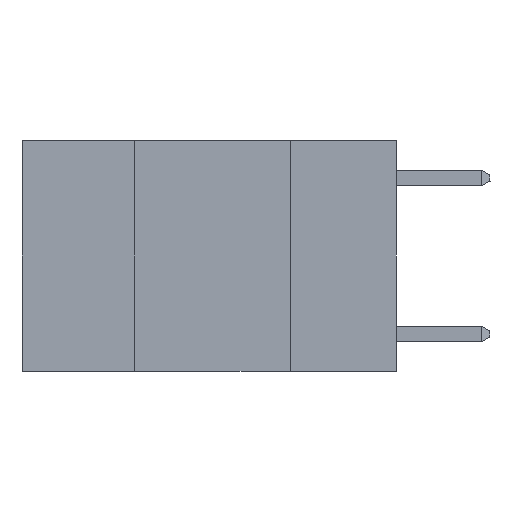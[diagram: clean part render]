
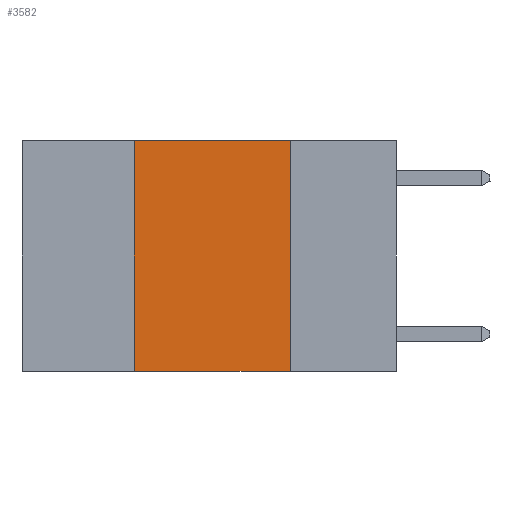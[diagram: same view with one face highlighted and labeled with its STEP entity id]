
A CAD part, left-side view. The second image highlights one B-rep face of the part: STEP entity #3582.
In plain terms, the highlighted planar face has unit normal (-1, 0, 0).
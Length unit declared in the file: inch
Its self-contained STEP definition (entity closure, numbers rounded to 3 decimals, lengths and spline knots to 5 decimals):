
#300 = DIRECTION ( 'NONE',  ( 0., -1., 0. ) ) ;
#587 = FACE_OUTER_BOUND ( 'NONE', #14649, .T. ) ;
#629 = AXIS2_PLACEMENT_3D ( 'NONE', #3977, #5288, #14118 ) ;
#1463 = LINE ( 'NONE', #1867, #2280 ) ;
#1574 = CARTESIAN_POINT ( 'NONE',  ( 0., 0.17, 0. ) ) ;
#1658 = VECTOR ( 'NONE', #9283, 39.37008 ) ;
#1867 = CARTESIAN_POINT ( 'NONE',  ( 0., 0.6, -0.37 ) ) ;
#2241 = LINE ( 'NONE', #16173, #15320 ) ;
#2280 = VECTOR ( 'NONE', #10849, 39.37008 ) ;
#2402 = VERTEX_POINT ( 'NONE', #11813 ) ;
#2422 = EDGE_CURVE ( 'NONE', #2402, #5420, #4739, .T. ) ;
#3582 = ADVANCED_FACE ( 'NONE', ( #587 ), #14069, .F. ) ;
#3977 = CARTESIAN_POINT ( 'NONE',  ( 0., 0.6, 0. ) ) ;
#4165 = CARTESIAN_POINT ( 'NONE',  ( 0., 0.42, 0. ) ) ;
#4739 = LINE ( 'NONE', #4165, #1658 ) ;
#5288 = DIRECTION ( 'NONE',  ( 1., 0., 0. ) ) ;
#5302 = CARTESIAN_POINT ( 'NONE',  ( 0., 0.42, 0. ) ) ;
#5420 = VERTEX_POINT ( 'NONE', #5302 ) ;
#6089 = LINE ( 'NONE', #9290, #15658 ) ;
#6255 = VERTEX_POINT ( 'NONE', #13141 ) ;
#6276 = DIRECTION ( 'NONE',  ( 0., 0., -1. ) ) ;
#8712 = EDGE_CURVE ( 'NONE', #16042, #6255, #2241, .T. ) ;
#9283 = DIRECTION ( 'NONE',  ( 0., 0., 1. ) ) ;
#9290 = CARTESIAN_POINT ( 'NONE',  ( 0., 0.6, 0. ) ) ;
#9646 = EDGE_CURVE ( 'NONE', #5420, #16042, #6089, .T. ) ;
#10849 = DIRECTION ( 'NONE',  ( 0., -1., 0. ) ) ;
#11813 = CARTESIAN_POINT ( 'NONE',  ( 0., 0.42, -0.37 ) ) ;
#12504 = ORIENTED_EDGE ( 'NONE', *, *, #8712, .F. ) ;
#13022 = EDGE_CURVE ( 'NONE', #2402, #6255, #1463, .T. ) ;
#13141 = CARTESIAN_POINT ( 'NONE',  ( 0., 0.17, -0.37 ) ) ;
#13853 = ORIENTED_EDGE ( 'NONE', *, *, #9646, .F. ) ;
#14069 = PLANE ( 'NONE',  #629 ) ;
#14118 = DIRECTION ( 'NONE',  ( 0., 0., -1. ) ) ;
#14649 = EDGE_LOOP ( 'NONE', ( #12504, #13853, #14836, #15172 ) ) ;
#14836 = ORIENTED_EDGE ( 'NONE', *, *, #2422, .F. ) ;
#15172 = ORIENTED_EDGE ( 'NONE', *, *, #13022, .T. ) ;
#15320 = VECTOR ( 'NONE', #6276, 39.37008 ) ;
#15658 = VECTOR ( 'NONE', #300, 39.37008 ) ;
#16042 = VERTEX_POINT ( 'NONE', #1574 ) ;
#16173 = CARTESIAN_POINT ( 'NONE',  ( 0., 0.17, 0. ) ) ;
